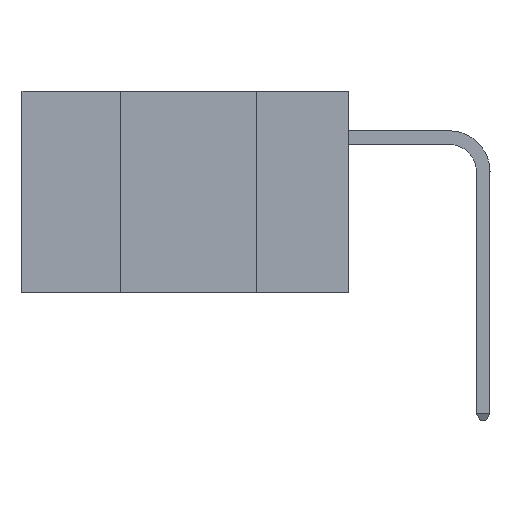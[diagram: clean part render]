
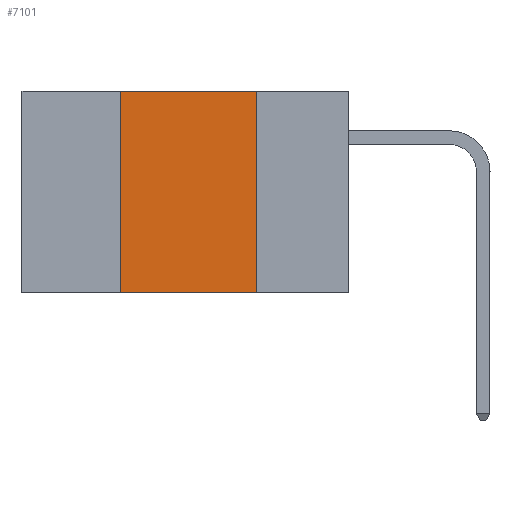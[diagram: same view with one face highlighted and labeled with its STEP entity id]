
A CAD part, left-side view. The second image highlights one B-rep face of the part: STEP entity #7101.
In plain terms, the highlighted planar face has unit normal (-1, 0, 0).
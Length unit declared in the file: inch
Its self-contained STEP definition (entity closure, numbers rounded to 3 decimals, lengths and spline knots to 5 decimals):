
#2271 = VECTOR ( 'NONE', #8971, 39.37008 ) ;
#4522 = DIRECTION ( 'NONE',  ( 0., 0., -1. ) ) ;
#5059 = VECTOR ( 'NONE', #7844, 39.37008 ) ;
#6491 = PLANE ( 'NONE',  #25619 ) ;
#6735 = CARTESIAN_POINT ( 'NONE',  ( 0., 0.17, 0. ) ) ;
#7101 = ADVANCED_FACE ( 'NONE', ( #18191 ), #6491, .F. ) ;
#7609 = ORIENTED_EDGE ( 'NONE', *, *, #10108, .F. ) ;
#7844 = DIRECTION ( 'NONE',  ( 0., -1., 0. ) ) ;
#8833 = CARTESIAN_POINT ( 'NONE',  ( 0., 0.17, 0. ) ) ;
#8971 = DIRECTION ( 'NONE',  ( 0., -1., 0. ) ) ;
#10108 = EDGE_CURVE ( 'NONE', #27660, #18562, #12012, .T. ) ;
#12012 = LINE ( 'NONE', #18955, #5059 ) ;
#13837 = EDGE_CURVE ( 'NONE', #18562, #19551, #21147, .T. ) ;
#14203 = ORIENTED_EDGE ( 'NONE', *, *, #15535, .F. ) ;
#15004 = VECTOR ( 'NONE', #29794, 39.37008 ) ;
#15535 = EDGE_CURVE ( 'NONE', #23570, #27660, #20424, .T. ) ;
#15868 = DIRECTION ( 'NONE',  ( 1., 0., 0. ) ) ;
#17619 = ORIENTED_EDGE ( 'NONE', *, *, #22593, .T. ) ;
#17819 = CARTESIAN_POINT ( 'NONE',  ( 0., 0.42, 0. ) ) ;
#18075 = CARTESIAN_POINT ( 'NONE',  ( 0., 0.6, -0.37 ) ) ;
#18191 = FACE_OUTER_BOUND ( 'NONE', #26735, .T. ) ;
#18365 = CARTESIAN_POINT ( 'NONE',  ( 0., 0.17, -0.37 ) ) ;
#18562 = VERTEX_POINT ( 'NONE', #6735 ) ;
#18955 = CARTESIAN_POINT ( 'NONE',  ( 0., 0.6, 0. ) ) ;
#19551 = VERTEX_POINT ( 'NONE', #18365 ) ;
#20424 = LINE ( 'NONE', #17819, #15004 ) ;
#21139 = ORIENTED_EDGE ( 'NONE', *, *, #13837, .F. ) ;
#21147 = LINE ( 'NONE', #8833, #21919 ) ;
#21919 = VECTOR ( 'NONE', #4522, 39.37008 ) ;
#22500 = CARTESIAN_POINT ( 'NONE',  ( 0., 0.6, 0. ) ) ;
#22593 = EDGE_CURVE ( 'NONE', #23570, #19551, #30208, .T. ) ;
#23535 = CARTESIAN_POINT ( 'NONE',  ( 0., 0.42, 0. ) ) ;
#23570 = VERTEX_POINT ( 'NONE', #25392 ) ;
#25091 = DIRECTION ( 'NONE',  ( 0., 0., -1. ) ) ;
#25392 = CARTESIAN_POINT ( 'NONE',  ( 0., 0.42, -0.37 ) ) ;
#25619 = AXIS2_PLACEMENT_3D ( 'NONE', #22500, #15868, #25091 ) ;
#26735 = EDGE_LOOP ( 'NONE', ( #21139, #7609, #14203, #17619 ) ) ;
#27660 = VERTEX_POINT ( 'NONE', #23535 ) ;
#29794 = DIRECTION ( 'NONE',  ( 0., 0., 1. ) ) ;
#30208 = LINE ( 'NONE', #18075, #2271 ) ;
